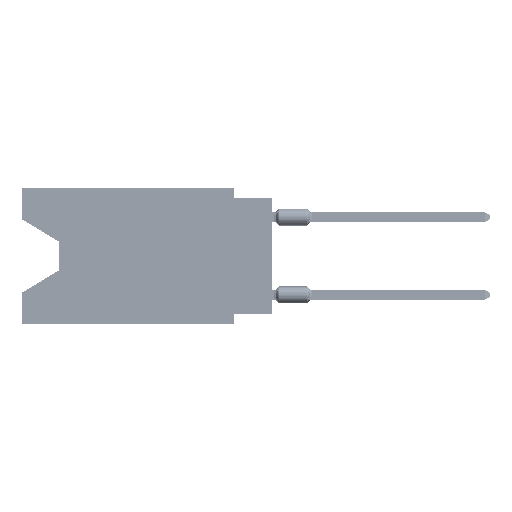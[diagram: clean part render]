
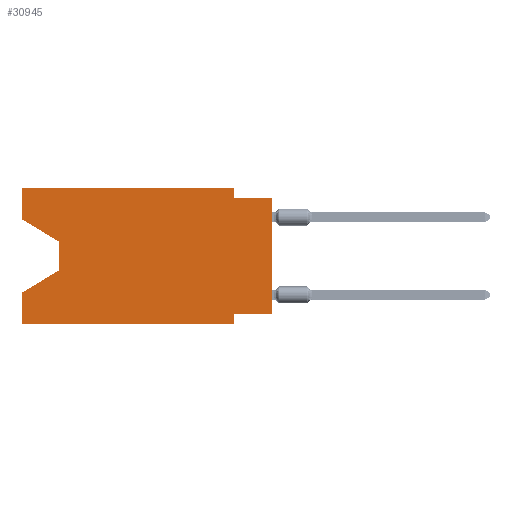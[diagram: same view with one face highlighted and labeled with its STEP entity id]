
A CAD part, left-side view. The second image highlights one B-rep face of the part: STEP entity #30945.
In plain terms, the highlighted planar face has unit normal (-1, 0, 0).
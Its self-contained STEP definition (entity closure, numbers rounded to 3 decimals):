
#147 = VERTEX_POINT ( 'NONE', #56700 ) ;
#2801 = LINE ( 'NONE', #86118, #66502 ) ;
#3334 = LINE ( 'NONE', #40467, #5288 ) ;
#5278 = VECTOR ( 'NONE', #112928, 1000. ) ;
#5288 = VECTOR ( 'NONE', #77541, 1000. ) ;
#6151 = AXIS2_PLACEMENT_3D ( 'NONE', #118581, #52935, #45195 ) ;
#6188 = CARTESIAN_POINT ( 'NONE',  ( 0., 16.383, 0. ) ) ;
#6599 = VERTEX_POINT ( 'NONE', #37115 ) ;
#6672 = LINE ( 'NONE', #51701, #100799 ) ;
#7952 = DIRECTION ( 'NONE',  ( 0., 0.855, -0.519 ) ) ;
#8513 = VERTEX_POINT ( 'NONE', #117289 ) ;
#9306 = ORIENTED_EDGE ( 'NONE', *, *, #111189, .F. ) ;
#10880 = DIRECTION ( 'NONE',  ( 0., 0., 1. ) ) ;
#13753 = CARTESIAN_POINT ( 'NONE',  ( 0., 0., -8.255 ) ) ;
#14173 = DIRECTION ( 'NONE',  ( 0., 0., -1. ) ) ;
#18105 = CARTESIAN_POINT ( 'NONE',  ( 0., 16.383, -8.89 ) ) ;
#19903 = LINE ( 'NONE', #18105, #5278 ) ;
#21180 = CARTESIAN_POINT ( 'NONE',  ( 0., 16.383, 0. ) ) ;
#23343 = ORIENTED_EDGE ( 'NONE', *, *, #72003, .F. ) ;
#25542 = DIRECTION ( 'NONE',  ( 0., 0., 1. ) ) ;
#27889 = ORIENTED_EDGE ( 'NONE', *, *, #34744, .F. ) ;
#28082 = EDGE_CURVE ( 'NONE', #44343, #71815, #64538, .T. ) ;
#29751 = LINE ( 'NONE', #66828, #43087 ) ;
#30945 = ADVANCED_FACE ( 'NONE', ( #91793 ), #71771, .F. ) ;
#31090 = EDGE_CURVE ( 'NONE', #32503, #50121, #29751, .T. ) ;
#31224 = ORIENTED_EDGE ( 'NONE', *, *, #96394, .T. ) ;
#31630 = VECTOR ( 'NONE', #7952, 1000. ) ;
#32431 = LINE ( 'NONE', #69509, #40763 ) ;
#32503 = VERTEX_POINT ( 'NONE', #83572 ) ;
#34744 = EDGE_CURVE ( 'NONE', #100747, #69111, #95847, .T. ) ;
#35820 = VECTOR ( 'NONE', #50248, 1000. ) ;
#36431 = EDGE_CURVE ( 'NONE', #147, #8513, #75293, .T. ) ;
#37115 = CARTESIAN_POINT ( 'NONE',  ( 0., 13.97, -3.505 ) ) ;
#40467 = CARTESIAN_POINT ( 'NONE',  ( 0., 16.383, -2.038 ) ) ;
#40763 = VECTOR ( 'NONE', #14173, 1000. ) ;
#43004 = ORIENTED_EDGE ( 'NONE', *, *, #64554, .T. ) ;
#43087 = VECTOR ( 'NONE', #10880, 1000. ) ;
#43661 = CARTESIAN_POINT ( 'NONE',  ( 0., 16.383, -6.852 ) ) ;
#44343 = VERTEX_POINT ( 'NONE', #57072 ) ;
#45195 = DIRECTION ( 'NONE',  ( 0., 0., -1. ) ) ;
#48379 = CARTESIAN_POINT ( 'NONE',  ( 0., 2.54, 0. ) ) ;
#49226 = EDGE_CURVE ( 'NONE', #44343, #6599, #3334, .T. ) ;
#50021 = ORIENTED_EDGE ( 'NONE', *, *, #36431, .F. ) ;
#50121 = VERTEX_POINT ( 'NONE', #43661 ) ;
#50248 = DIRECTION ( 'NONE',  ( 0., 1., 0. ) ) ;
#51445 = CARTESIAN_POINT ( 'NONE',  ( 0., 0., -8.255 ) ) ;
#51701 = CARTESIAN_POINT ( 'NONE',  ( 0., 0., 0. ) ) ;
#52249 = ORIENTED_EDGE ( 'NONE', *, *, #31090, .F. ) ;
#52935 = DIRECTION ( 'NONE',  ( 1., 0., 0. ) ) ;
#53891 = ORIENTED_EDGE ( 'NONE', *, *, #49226, .T. ) ;
#55381 = CARTESIAN_POINT ( 'NONE',  ( 0., 13.97, -5.385 ) ) ;
#56700 = CARTESIAN_POINT ( 'NONE',  ( 0., 2.54, -0.635 ) ) ;
#57072 = CARTESIAN_POINT ( 'NONE',  ( 0., 16.383, -2.038 ) ) ;
#57574 = DIRECTION ( 'NONE',  ( 0., 0., -1. ) ) ;
#57826 = VERTEX_POINT ( 'NONE', #48379 ) ;
#59876 = DIRECTION ( 'NONE',  ( 0., -1., 0. ) ) ;
#60042 = VECTOR ( 'NONE', #86857, 1000. ) ;
#63067 = CARTESIAN_POINT ( 'NONE',  ( 0., 13.97, -5.385 ) ) ;
#63328 = LINE ( 'NONE', #55381, #31630 ) ;
#64538 = LINE ( 'NONE', #6188, #116326 ) ;
#64554 = EDGE_CURVE ( 'NONE', #66621, #50121, #63328, .T. ) ;
#66502 = VECTOR ( 'NONE', #57574, 1000. ) ;
#66621 = VERTEX_POINT ( 'NONE', #63067 ) ;
#66828 = CARTESIAN_POINT ( 'NONE',  ( 0., 16.383, 0. ) ) ;
#69111 = VERTEX_POINT ( 'NONE', #100019 ) ;
#69177 = ORIENTED_EDGE ( 'NONE', *, *, #28082, .F. ) ;
#69509 = CARTESIAN_POINT ( 'NONE',  ( 0., 2.54, -8.89 ) ) ;
#70392 = VERTEX_POINT ( 'NONE', #75940 ) ;
#71771 = PLANE ( 'NONE',  #6151 ) ;
#71815 = VERTEX_POINT ( 'NONE', #108997 ) ;
#72003 = EDGE_CURVE ( 'NONE', #57826, #147, #2801, .T. ) ;
#74696 = CARTESIAN_POINT ( 'NONE',  ( 0., 0., -0.635 ) ) ;
#74945 = VECTOR ( 'NONE', #59876, 1000. ) ;
#75293 = LINE ( 'NONE', #74696, #74945 ) ;
#75940 = CARTESIAN_POINT ( 'NONE',  ( 0., 2.54, -8.89 ) ) ;
#77086 = EDGE_LOOP ( 'NONE', ( #53891, #97392, #43004, #52249, #31224, #78891, #27889, #114788, #50021, #23343, #9306, #69177 ) ) ;
#77541 = DIRECTION ( 'NONE',  ( 0., -0.855, -0.519 ) ) ;
#78891 = ORIENTED_EDGE ( 'NONE', *, *, #114683, .F. ) ;
#83572 = CARTESIAN_POINT ( 'NONE',  ( 0., 16.383, -8.89 ) ) ;
#86118 = CARTESIAN_POINT ( 'NONE',  ( 0., 2.54, 0. ) ) ;
#86225 = DIRECTION ( 'NONE',  ( 0., -1., 0. ) ) ;
#86857 = DIRECTION ( 'NONE',  ( 0., 0., -1. ) ) ;
#89275 = EDGE_CURVE ( 'NONE', #100747, #8513, #6672, .T. ) ;
#90110 = DIRECTION ( 'NONE',  ( 0., 0., 1. ) ) ;
#91793 = FACE_OUTER_BOUND ( 'NONE', #77086, .T. ) ;
#95339 = LINE ( 'NONE', #21180, #113944 ) ;
#95847 = LINE ( 'NONE', #13753, #35820 ) ;
#96394 = EDGE_CURVE ( 'NONE', #32503, #70392, #19903, .T. ) ;
#97392 = ORIENTED_EDGE ( 'NONE', *, *, #98572, .T. ) ;
#98572 = EDGE_CURVE ( 'NONE', #6599, #66621, #106313, .T. ) ;
#100019 = CARTESIAN_POINT ( 'NONE',  ( 0., 2.54, -8.255 ) ) ;
#100747 = VERTEX_POINT ( 'NONE', #51445 ) ;
#100799 = VECTOR ( 'NONE', #25542, 1000. ) ;
#106313 = LINE ( 'NONE', #113649, #60042 ) ;
#108997 = CARTESIAN_POINT ( 'NONE',  ( 0., 16.383, 0. ) ) ;
#111189 = EDGE_CURVE ( 'NONE', #71815, #57826, #95339, .T. ) ;
#112928 = DIRECTION ( 'NONE',  ( 0., -1., 0. ) ) ;
#113649 = CARTESIAN_POINT ( 'NONE',  ( 0., 13.97, -3.505 ) ) ;
#113944 = VECTOR ( 'NONE', #86225, 1000. ) ;
#114683 = EDGE_CURVE ( 'NONE', #69111, #70392, #32431, .T. ) ;
#114788 = ORIENTED_EDGE ( 'NONE', *, *, #89275, .T. ) ;
#116326 = VECTOR ( 'NONE', #90110, 1000. ) ;
#117289 = CARTESIAN_POINT ( 'NONE',  ( 0., 0., -0.635 ) ) ;
#118581 = CARTESIAN_POINT ( 'NONE',  ( 0., 16.383, 0. ) ) ;
